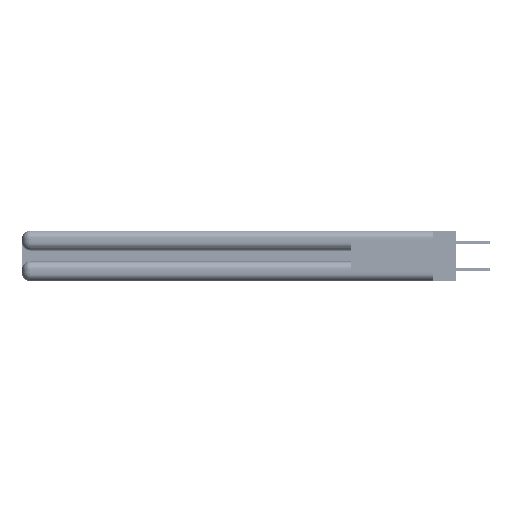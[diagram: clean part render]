
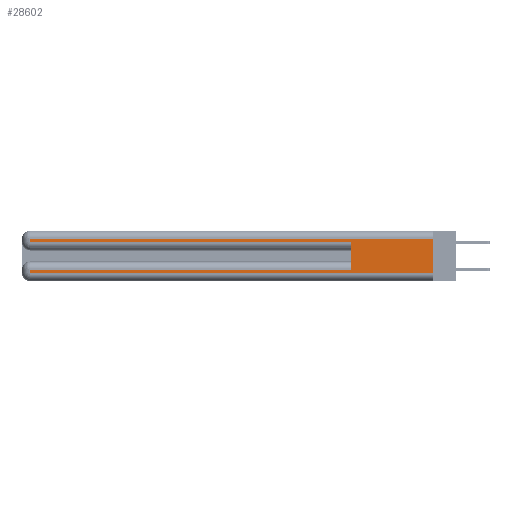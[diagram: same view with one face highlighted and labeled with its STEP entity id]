
A CAD part, left-side view. The second image highlights one B-rep face of the part: STEP entity #28602.
In plain terms, the highlighted planar face has unit normal (-1, 0, 0).
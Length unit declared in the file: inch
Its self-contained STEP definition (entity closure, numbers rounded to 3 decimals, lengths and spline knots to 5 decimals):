
#1036 = ORIENTED_EDGE ( 'NONE', *, *, #1649, .T. ) ;
#1061 = VERTEX_POINT ( 'NONE', #45327 ) ;
#1649 = EDGE_CURVE ( 'NONE', #33636, #1061, #41044, .T. ) ;
#1672 = LINE ( 'NONE', #31336, #37827 ) ;
#2344 = VERTEX_POINT ( 'NONE', #19370 ) ;
#5208 = DIRECTION ( 'NONE',  ( 1., 0., 0. ) ) ;
#5540 = LINE ( 'NONE', #37712, #44188 ) ;
#7292 = DIRECTION ( 'NONE',  ( 0., -1., 0. ) ) ;
#8425 = EDGE_CURVE ( 'NONE', #21089, #33636, #30325, .T. ) ;
#9230 = EDGE_CURVE ( 'NONE', #2344, #10215, #32070, .T. ) ;
#9538 = EDGE_CURVE ( 'NONE', #12996, #19560, #5540, .T. ) ;
#10215 = VERTEX_POINT ( 'NONE', #30985 ) ;
#10367 = ORIENTED_EDGE ( 'NONE', *, *, #8425, .T. ) ;
#11015 = CARTESIAN_POINT ( 'NONE',  ( 0., 2.94, 0.31 ) ) ;
#12199 = CARTESIAN_POINT ( 'NONE',  ( 0., 0., 0.37 ) ) ;
#12502 = DIRECTION ( 'NONE',  ( 0., 1., 0. ) ) ;
#12961 = LINE ( 'NONE', #17213, #43747 ) ;
#12996 = VERTEX_POINT ( 'NONE', #24914 ) ;
#14748 = ORIENTED_EDGE ( 'NONE', *, *, #9538, .T. ) ;
#15643 = DIRECTION ( 'NONE',  ( 0., 0., -1. ) ) ;
#16318 = CARTESIAN_POINT ( 'NONE',  ( 0., 2.94, 0.285 ) ) ;
#16349 = EDGE_LOOP ( 'NONE', ( #36060, #22520, #10367, #1036, #44030, #14748, #44445, #29909 ) ) ;
#16549 = DIRECTION ( 'NONE',  ( 0., 0., -1. ) ) ;
#16675 = VERTEX_POINT ( 'NONE', #47339 ) ;
#17213 = CARTESIAN_POINT ( 'NONE',  ( 0., 2.94, 0.37 ) ) ;
#18310 = VECTOR ( 'NONE', #15643, 39.37008 ) ;
#18497 = DIRECTION ( 'NONE',  ( 0., 1., 0. ) ) ;
#19092 = CARTESIAN_POINT ( 'NONE',  ( 0., 2.94, 0.085 ) ) ;
#19370 = CARTESIAN_POINT ( 'NONE',  ( 0., 0., 0.31 ) ) ;
#19560 = VERTEX_POINT ( 'NONE', #19092 ) ;
#20535 = PLANE ( 'NONE',  #35194 ) ;
#21089 = VERTEX_POINT ( 'NONE', #11015 ) ;
#21402 = DIRECTION ( 'NONE',  ( 0., 0., 1. ) ) ;
#21820 = VECTOR ( 'NONE', #39819, 39.37008 ) ;
#22520 = ORIENTED_EDGE ( 'NONE', *, *, #23963, .T. ) ;
#23963 = EDGE_CURVE ( 'NONE', #2344, #21089, #48282, .T. ) ;
#24558 = DIRECTION ( 'NONE',  ( 0., 0., -1. ) ) ;
#24914 = CARTESIAN_POINT ( 'NONE',  ( 0., 0.6, 0.085 ) ) ;
#26331 = CARTESIAN_POINT ( 'NONE',  ( 0., 0., 0.285 ) ) ;
#27145 = VECTOR ( 'NONE', #12502, 39.37008 ) ;
#28309 = CARTESIAN_POINT ( 'NONE',  ( 0., 0., 0.31 ) ) ;
#28602 = ADVANCED_FACE ( 'NONE', ( #32827 ), #20535, .F. ) ;
#29909 = ORIENTED_EDGE ( 'NONE', *, *, #43600, .T. ) ;
#30325 = LINE ( 'NONE', #42294, #18310 ) ;
#30582 = VECTOR ( 'NONE', #35284, 39.37008 ) ;
#30985 = CARTESIAN_POINT ( 'NONE',  ( 0., 0., 0.06 ) ) ;
#31336 = CARTESIAN_POINT ( 'NONE',  ( 0., 0.6, 0.145 ) ) ;
#32070 = LINE ( 'NONE', #12199, #21820 ) ;
#32827 = FACE_OUTER_BOUND ( 'NONE', #16349, .T. ) ;
#33636 = VERTEX_POINT ( 'NONE', #16318 ) ;
#35194 = AXIS2_PLACEMENT_3D ( 'NONE', #47225, #5208, #24558 ) ;
#35284 = DIRECTION ( 'NONE',  ( 0., -1., 0. ) ) ;
#36060 = ORIENTED_EDGE ( 'NONE', *, *, #9230, .F. ) ;
#37712 = CARTESIAN_POINT ( 'NONE',  ( 0., 0., 0.085 ) ) ;
#37827 = VECTOR ( 'NONE', #21402, 39.37008 ) ;
#39149 = CARTESIAN_POINT ( 'NONE',  ( 0., 0., 0.06 ) ) ;
#39178 = VECTOR ( 'NONE', #7292, 39.37008 ) ;
#39205 = EDGE_CURVE ( 'NONE', #19560, #16675, #12961, .T. ) ;
#39819 = DIRECTION ( 'NONE',  ( 0., 0., -1. ) ) ;
#41044 = LINE ( 'NONE', #26331, #39178 ) ;
#42294 = CARTESIAN_POINT ( 'NONE',  ( 0., 2.94, 0.37 ) ) ;
#43600 = EDGE_CURVE ( 'NONE', #16675, #10215, #48745, .T. ) ;
#43747 = VECTOR ( 'NONE', #16549, 39.37008 ) ;
#43931 = EDGE_CURVE ( 'NONE', #12996, #1061, #1672, .T. ) ;
#44030 = ORIENTED_EDGE ( 'NONE', *, *, #43931, .F. ) ;
#44188 = VECTOR ( 'NONE', #18497, 39.37008 ) ;
#44445 = ORIENTED_EDGE ( 'NONE', *, *, #39205, .T. ) ;
#45327 = CARTESIAN_POINT ( 'NONE',  ( 0., 0.6, 0.285 ) ) ;
#47225 = CARTESIAN_POINT ( 'NONE',  ( 0., 0., 0.37 ) ) ;
#47339 = CARTESIAN_POINT ( 'NONE',  ( 0., 2.94, 0.06 ) ) ;
#48282 = LINE ( 'NONE', #28309, #27145 ) ;
#48745 = LINE ( 'NONE', #39149, #30582 ) ;
